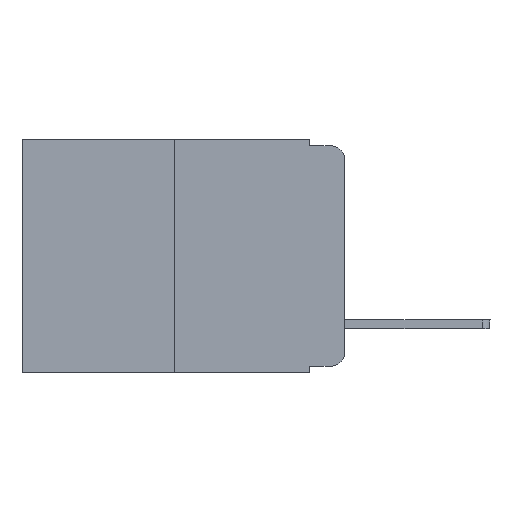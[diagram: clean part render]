
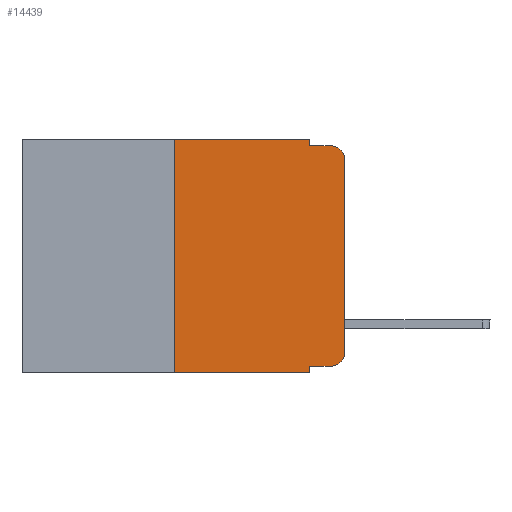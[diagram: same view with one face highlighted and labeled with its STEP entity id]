
A CAD part, left-side view. The second image highlights one B-rep face of the part: STEP entity #14439.
In plain terms, the highlighted planar face has unit normal (-1, 0, 0).
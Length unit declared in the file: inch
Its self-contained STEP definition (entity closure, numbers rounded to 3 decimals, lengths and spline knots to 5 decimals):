
#81 = VECTOR ( 'NONE', #6423, 39.37008 ) ;
#89 = CARTESIAN_POINT ( 'NONE',  ( 0., 0.02, -0.01 ) ) ;
#149 = VERTEX_POINT ( 'NONE', #189 ) ;
#189 = CARTESIAN_POINT ( 'NONE',  ( 0., 0., -0.313 ) ) ;
#240 = LINE ( 'NONE', #16173, #13595 ) ;
#669 = LINE ( 'NONE', #17035, #2577 ) ;
#934 = CIRCLE ( 'NONE', #10399, 0.02 ) ;
#1000 = VERTEX_POINT ( 'NONE', #17647 ) ;
#1101 = CARTESIAN_POINT ( 'NONE',  ( 0., 0.02, -0.313 ) ) ;
#1151 = LINE ( 'NONE', #13367, #81 ) ;
#1214 = ORIENTED_EDGE ( 'NONE', *, *, #16798, .T. ) ;
#1336 = AXIS2_PLACEMENT_3D ( 'NONE', #19156, #22362, #3638 ) ;
#1482 = DIRECTION ( 'NONE',  ( 0., 0., -1. ) ) ;
#1500 = LINE ( 'NONE', #21852, #14803 ) ;
#1708 = VECTOR ( 'NONE', #8629, 39.37008 ) ;
#1865 = ORIENTED_EDGE ( 'NONE', *, *, #6918, .F. ) ;
#2405 = VERTEX_POINT ( 'NONE', #8988 ) ;
#2418 = CARTESIAN_POINT ( 'NONE',  ( 0., 0.25, 0. ) ) ;
#2554 = LINE ( 'NONE', #12398, #19645 ) ;
#2577 = VECTOR ( 'NONE', #1482, 39.37008 ) ;
#3251 = VERTEX_POINT ( 'NONE', #2418 ) ;
#3370 = FACE_OUTER_BOUND ( 'NONE', #6108, .T. ) ;
#3610 = LINE ( 'NONE', #13198, #4666 ) ;
#3638 = DIRECTION ( 'NONE',  ( 0., 0., -1. ) ) ;
#3924 = EDGE_CURVE ( 'NONE', #2405, #8519, #240, .T. ) ;
#4041 = CARTESIAN_POINT ( 'NONE',  ( 0., 0.051, -0.343 ) ) ;
#4521 = VERTEX_POINT ( 'NONE', #16574 ) ;
#4666 = VECTOR ( 'NONE', #9838, 39.37008 ) ;
#4709 = DIRECTION ( 'NONE',  ( 0., 0., -1. ) ) ;
#4738 = VERTEX_POINT ( 'NONE', #17550 ) ;
#5132 = CARTESIAN_POINT ( 'NONE',  ( 0., 0.473, 0. ) ) ;
#5162 = CARTESIAN_POINT ( 'NONE',  ( 0., 0.051, -0.333 ) ) ;
#5199 = PLANE ( 'NONE',  #1336 ) ;
#6108 = EDGE_LOOP ( 'NONE', ( #16766, #1214, #18312, #14200, #9836, #16068, #20363, #1865, #14176, #21806 ) ) ;
#6423 = DIRECTION ( 'NONE',  ( 0., 0., 1. ) ) ;
#6918 = EDGE_CURVE ( 'NONE', #4521, #13416, #669, .T. ) ;
#7673 = DIRECTION ( 'NONE',  ( 0., -1., 0. ) ) ;
#8519 = VERTEX_POINT ( 'NONE', #89 ) ;
#8629 = DIRECTION ( 'NONE',  ( 0., -1., 0. ) ) ;
#8988 = CARTESIAN_POINT ( 'NONE',  ( 0., 0.051, -0.01 ) ) ;
#9165 = EDGE_CURVE ( 'NONE', #4738, #3251, #1151, .T. ) ;
#9277 = CARTESIAN_POINT ( 'NONE',  ( 0., 0.051, 0. ) ) ;
#9836 = ORIENTED_EDGE ( 'NONE', *, *, #14364, .F. ) ;
#9838 = DIRECTION ( 'NONE',  ( 0., 0., -1. ) ) ;
#10399 = AXIS2_PLACEMENT_3D ( 'NONE', #15132, #13559, #4709 ) ;
#10457 = EDGE_CURVE ( 'NONE', #12558, #149, #17396, .T. ) ;
#11684 = DIRECTION ( 'NONE',  ( 0., 0., -1. ) ) ;
#12398 = CARTESIAN_POINT ( 'NONE',  ( 0., 0., 0. ) ) ;
#12558 = VERTEX_POINT ( 'NONE', #18722 ) ;
#13198 = CARTESIAN_POINT ( 'NONE',  ( 0., 0.051, 0. ) ) ;
#13367 = CARTESIAN_POINT ( 'NONE',  ( 0., 0.25, 0. ) ) ;
#13416 = VERTEX_POINT ( 'NONE', #4041 ) ;
#13559 = DIRECTION ( 'NONE',  ( -1., 0., 0. ) ) ;
#13595 = VECTOR ( 'NONE', #7673, 39.37008 ) ;
#13698 = EDGE_CURVE ( 'NONE', #4521, #12558, #15859, .T. ) ;
#13883 = EDGE_CURVE ( 'NONE', #149, #1000, #2554, .T. ) ;
#14176 = ORIENTED_EDGE ( 'NONE', *, *, #13698, .T. ) ;
#14200 = ORIENTED_EDGE ( 'NONE', *, *, #22045, .F. ) ;
#14364 = EDGE_CURVE ( 'NONE', #3251, #22400, #21791, .T. ) ;
#14439 = ADVANCED_FACE ( 'NONE', ( #3370 ), #5199, .F. ) ;
#14803 = VECTOR ( 'NONE', #15039, 39.37008 ) ;
#15039 = DIRECTION ( 'NONE',  ( 0., -1., 0. ) ) ;
#15132 = CARTESIAN_POINT ( 'NONE',  ( 0., 0.02, -0.03 ) ) ;
#15715 = DIRECTION ( 'NONE',  ( 0., 0., 1. ) ) ;
#15859 = LINE ( 'NONE', #5162, #21842 ) ;
#16068 = ORIENTED_EDGE ( 'NONE', *, *, #9165, .F. ) ;
#16173 = CARTESIAN_POINT ( 'NONE',  ( 0., 0.051, -0.01 ) ) ;
#16574 = CARTESIAN_POINT ( 'NONE',  ( 0., 0.051, -0.333 ) ) ;
#16766 = ORIENTED_EDGE ( 'NONE', *, *, #13883, .T. ) ;
#16798 = EDGE_CURVE ( 'NONE', #1000, #8519, #934, .T. ) ;
#16898 = DIRECTION ( 'NONE',  ( -1., 0., 0. ) ) ;
#17035 = CARTESIAN_POINT ( 'NONE',  ( 0., 0.051, 0. ) ) ;
#17396 = CIRCLE ( 'NONE', #17897, 0.02 ) ;
#17550 = CARTESIAN_POINT ( 'NONE',  ( 0., 0.25, -0.343 ) ) ;
#17647 = CARTESIAN_POINT ( 'NONE',  ( 0., 0., -0.03 ) ) ;
#17897 = AXIS2_PLACEMENT_3D ( 'NONE', #1101, #16898, #11684 ) ;
#18312 = ORIENTED_EDGE ( 'NONE', *, *, #3924, .F. ) ;
#18722 = CARTESIAN_POINT ( 'NONE',  ( 0., 0.02, -0.333 ) ) ;
#18826 = DIRECTION ( 'NONE',  ( 0., -1., 0. ) ) ;
#19156 = CARTESIAN_POINT ( 'NONE',  ( 0., 0.473, 0. ) ) ;
#19645 = VECTOR ( 'NONE', #15715, 39.37008 ) ;
#20363 = ORIENTED_EDGE ( 'NONE', *, *, #20580, .T. ) ;
#20580 = EDGE_CURVE ( 'NONE', #4738, #13416, #1500, .T. ) ;
#21791 = LINE ( 'NONE', #5132, #1708 ) ;
#21806 = ORIENTED_EDGE ( 'NONE', *, *, #10457, .T. ) ;
#21842 = VECTOR ( 'NONE', #18826, 39.37008 ) ;
#21852 = CARTESIAN_POINT ( 'NONE',  ( 0., 0.473, -0.343 ) ) ;
#22045 = EDGE_CURVE ( 'NONE', #22400, #2405, #3610, .T. ) ;
#22362 = DIRECTION ( 'NONE',  ( 1., 0., 0. ) ) ;
#22400 = VERTEX_POINT ( 'NONE', #9277 ) ;
